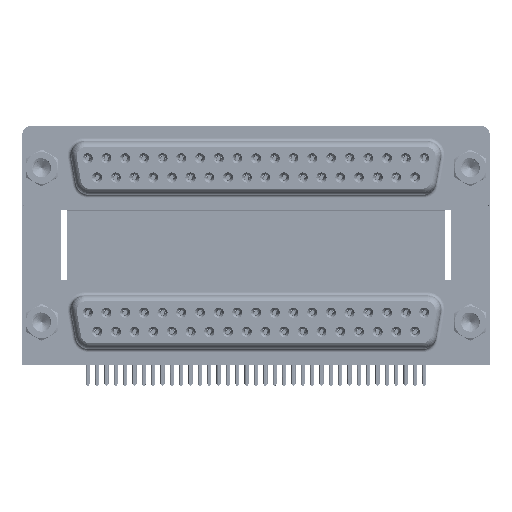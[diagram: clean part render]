
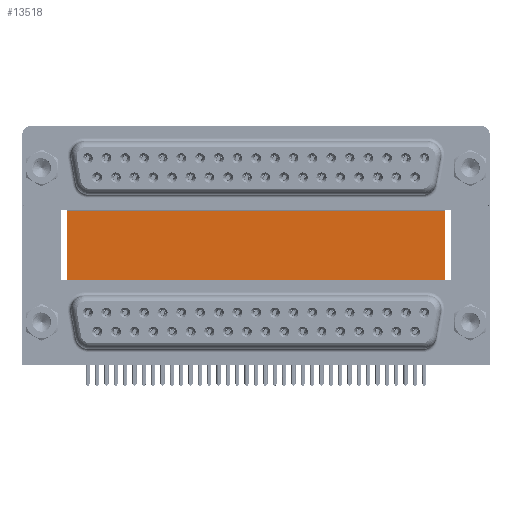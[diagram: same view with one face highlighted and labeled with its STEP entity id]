
A CAD part, top view. The second image highlights one B-rep face of the part: STEP entity #13518.
In plain terms, the highlighted planar face has unit normal (0, 0, 1).
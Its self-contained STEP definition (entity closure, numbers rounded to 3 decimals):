
#2719 = CARTESIAN_POINT ( 'NONE',  ( 3.79, -3.735, -12. ) ) ;
#4636 = EDGE_CURVE ( 'NONE', #58936, #47270, #39667, .T. ) ;
#5022 = CARTESIAN_POINT ( 'NONE',  ( 3.79, 16.585, -12. ) ) ;
#5824 = LINE ( 'NONE', #73158, #56150 ) ;
#6599 = DIRECTION ( 'NONE',  ( -1., 0., 0. ) ) ;
#7092 = LINE ( 'NONE', #56390, #45094 ) ;
#9619 = CARTESIAN_POINT ( 'NONE',  ( 59.71, -3.735, -12. ) ) ;
#13518 = ADVANCED_FACE ( 'NONE', ( #49106 ), #47926, .F. ) ;
#15470 = CARTESIAN_POINT ( 'NONE',  ( 3.79, 16.585, -12. ) ) ;
#29112 = EDGE_CURVE ( 'NONE', #58936, #49534, #45904, .T. ) ;
#35313 = ORIENTED_EDGE ( 'NONE', *, *, #4636, .F. ) ;
#36300 = DIRECTION ( 'NONE',  ( 0., 0., -1. ) ) ;
#36746 = ORIENTED_EDGE ( 'NONE', *, *, #76126, .T. ) ;
#39667 = LINE ( 'NONE', #63728, #49416 ) ;
#43109 = DIRECTION ( 'NONE',  ( 1., 0., 0. ) ) ;
#45094 = VECTOR ( 'NONE', #50773, 1000. ) ;
#45904 = LINE ( 'NONE', #15470, #56496 ) ;
#46075 = DIRECTION ( 'NONE',  ( 1., 0., 0. ) ) ;
#47270 = VERTEX_POINT ( 'NONE', #60590 ) ;
#47926 = PLANE ( 'NONE',  #79223 ) ;
#47957 = EDGE_LOOP ( 'NONE', ( #36746, #56075, #35313, #55749 ) ) ;
#49106 = FACE_OUTER_BOUND ( 'NONE', #47957, .T. ) ;
#49416 = VECTOR ( 'NONE', #46075, 1000. ) ;
#49534 = VERTEX_POINT ( 'NONE', #2719 ) ;
#50773 = DIRECTION ( 'NONE',  ( 0., -1., 0. ) ) ;
#55749 = ORIENTED_EDGE ( 'NONE', *, *, #29112, .T. ) ;
#56075 = ORIENTED_EDGE ( 'NONE', *, *, #69278, .F. ) ;
#56150 = VECTOR ( 'NONE', #43109, 1000. ) ;
#56390 = CARTESIAN_POINT ( 'NONE',  ( 59.71, 16.585, -12. ) ) ;
#56496 = VECTOR ( 'NONE', #59134, 1000. ) ;
#58936 = VERTEX_POINT ( 'NONE', #66502 ) ;
#59134 = DIRECTION ( 'NONE',  ( 0., -1., 0. ) ) ;
#60590 = CARTESIAN_POINT ( 'NONE',  ( 59.71, 16.585, -12. ) ) ;
#63728 = CARTESIAN_POINT ( 'NONE',  ( 3.79, 16.585, -12. ) ) ;
#66502 = CARTESIAN_POINT ( 'NONE',  ( 3.79, 16.585, -12. ) ) ;
#66618 = VERTEX_POINT ( 'NONE', #9619 ) ;
#69278 = EDGE_CURVE ( 'NONE', #47270, #66618, #7092, .T. ) ;
#73158 = CARTESIAN_POINT ( 'NONE',  ( 3.79, -3.735, -12. ) ) ;
#76126 = EDGE_CURVE ( 'NONE', #49534, #66618, #5824, .T. ) ;
#79223 = AXIS2_PLACEMENT_3D ( 'NONE', #5022, #36300, #6599 ) ;
